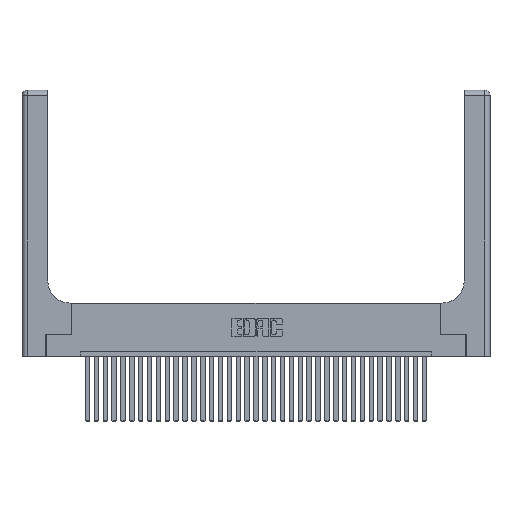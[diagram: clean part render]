
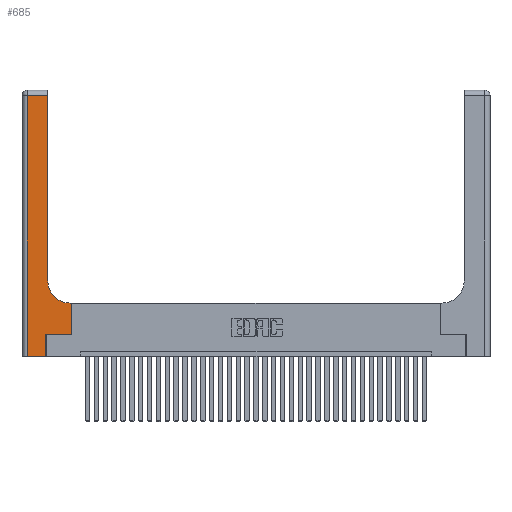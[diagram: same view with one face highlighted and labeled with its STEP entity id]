
A CAD part, top view. The second image highlights one B-rep face of the part: STEP entity #685.
In plain terms, the highlighted planar face has unit normal (0, 0, 1).
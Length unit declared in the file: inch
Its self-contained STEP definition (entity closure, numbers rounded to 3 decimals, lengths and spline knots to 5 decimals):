
#685 = ADVANCED_FACE ( 'NONE', ( #22974 ), #1935, .F. ) ;
#706 = DIRECTION ( 'NONE',  ( 1., 0., 0. ) ) ;
#1935 = PLANE ( 'NONE',  #8416 ) ;
#2700 = CARTESIAN_POINT ( 'NONE',  ( 0.269, 0.25, 0.37 ) ) ;
#2873 = VECTOR ( 'NONE', #17566, 39.37008 ) ;
#2950 = VECTOR ( 'NONE', #16315, 39.37008 ) ;
#4067 = CARTESIAN_POINT ( 'NONE',  ( 0.06, 2.94, 0.37 ) ) ;
#4298 = LINE ( 'NONE', #26759, #11896 ) ;
#4313 = LINE ( 'NONE', #32021, #24078 ) ;
#4725 = VERTEX_POINT ( 'NONE', #21585 ) ;
#5395 = VECTOR ( 'NONE', #26008, 39.37008 ) ;
#5499 = CARTESIAN_POINT ( 'NONE',  ( 0.269, 0., 0.37 ) ) ;
#6044 = VERTEX_POINT ( 'NONE', #33279 ) ;
#6497 = VERTEX_POINT ( 'NONE', #24967 ) ;
#6965 = EDGE_CURVE ( 'NONE', #30685, #6497, #4313, .T. ) ;
#8340 = EDGE_CURVE ( 'NONE', #4725, #32227, #15115, .T. ) ;
#8407 = ORIENTED_EDGE ( 'NONE', *, *, #8340, .T. ) ;
#8416 = AXIS2_PLACEMENT_3D ( 'NONE', #23293, #28463, #20472 ) ;
#8888 = EDGE_CURVE ( 'NONE', #29726, #4725, #24313, .T. ) ;
#9920 = ORIENTED_EDGE ( 'NONE', *, *, #10128, .T. ) ;
#10128 = EDGE_CURVE ( 'NONE', #32227, #30168, #34322, .T. ) ;
#10531 = VERTEX_POINT ( 'NONE', #11773 ) ;
#11012 = LINE ( 'NONE', #19578, #25315 ) ;
#11169 = DIRECTION ( 'NONE',  ( 1., 0., 0. ) ) ;
#11247 = ORIENTED_EDGE ( 'NONE', *, *, #6965, .T. ) ;
#11773 = CARTESIAN_POINT ( 'NONE',  ( 0.2915, 2.94, 0.37 ) ) ;
#11896 = VECTOR ( 'NONE', #32705, 39.37008 ) ;
#11966 = ORIENTED_EDGE ( 'NONE', *, *, #8888, .T. ) ;
#12348 = EDGE_LOOP ( 'NONE', ( #12729, #12396, #11247, #31427, #32516, #26527, #11966, #8407, #9920 ) ) ;
#12396 = ORIENTED_EDGE ( 'NONE', *, *, #17996, .T. ) ;
#12729 = ORIENTED_EDGE ( 'NONE', *, *, #33756, .T. ) ;
#12816 = CARTESIAN_POINT ( 'NONE',  ( 0.2915, 3., 0.37 ) ) ;
#13382 = DIRECTION ( 'NONE',  ( 0., 1., 0. ) ) ;
#13512 = CARTESIAN_POINT ( 'NONE',  ( 0.5415, 0.6, 0.37 ) ) ;
#14252 = CARTESIAN_POINT ( 'NONE',  ( 0.5585, 0.25, 0.37 ) ) ;
#14823 = VECTOR ( 'NONE', #13382, 39.37008 ) ;
#15115 = LINE ( 'NONE', #23066, #5395 ) ;
#16315 = DIRECTION ( 'NONE',  ( 0., 1., 0. ) ) ;
#17566 = DIRECTION ( 'NONE',  ( 0., 1., 0. ) ) ;
#17696 = CARTESIAN_POINT ( 'NONE',  ( 0.5585, 0.25, 0.37 ) ) ;
#17996 = EDGE_CURVE ( 'NONE', #10531, #30685, #4298, .T. ) ;
#19320 = LINE ( 'NONE', #5499, #2950 ) ;
#19557 = DIRECTION ( 'NONE',  ( 1., 0., 0. ) ) ;
#19578 = CARTESIAN_POINT ( 'NONE',  ( 0.269, 0.25, 0.37 ) ) ;
#19758 = CARTESIAN_POINT ( 'NONE',  ( 0.5415, 0.85, 0.37 ) ) ;
#19915 = EDGE_CURVE ( 'NONE', #6044, #21777, #19320, .T. ) ;
#20472 = DIRECTION ( 'NONE',  ( -1., 0., 0. ) ) ;
#20692 = LINE ( 'NONE', #32831, #21920 ) ;
#21003 = AXIS2_PLACEMENT_3D ( 'NONE', #19758, #26721, #11169 ) ;
#21585 = CARTESIAN_POINT ( 'NONE',  ( 0.5585, 0.6, 0.37 ) ) ;
#21777 = VERTEX_POINT ( 'NONE', #2700 ) ;
#21920 = VECTOR ( 'NONE', #19557, 39.37008 ) ;
#22329 = LINE ( 'NONE', #12816, #14823 ) ;
#22974 = FACE_OUTER_BOUND ( 'NONE', #12348, .T. ) ;
#23066 = CARTESIAN_POINT ( 'NONE',  ( 0.2915, 0.6, 0.37 ) ) ;
#23293 = CARTESIAN_POINT ( 'NONE',  ( 0., 3., 0.37 ) ) ;
#24078 = VECTOR ( 'NONE', #30248, 39.37008 ) ;
#24157 = EDGE_CURVE ( 'NONE', #21777, #29726, #11012, .T. ) ;
#24313 = LINE ( 'NONE', #17696, #2873 ) ;
#24967 = CARTESIAN_POINT ( 'NONE',  ( 0.06, 0., 0.37 ) ) ;
#25315 = VECTOR ( 'NONE', #706, 39.37008 ) ;
#26008 = DIRECTION ( 'NONE',  ( -1., 0., 0. ) ) ;
#26527 = ORIENTED_EDGE ( 'NONE', *, *, #24157, .T. ) ;
#26721 = DIRECTION ( 'NONE',  ( 0., 0., -1. ) ) ;
#26759 = CARTESIAN_POINT ( 'NONE',  ( 0., 2.94, 0.37 ) ) ;
#28463 = DIRECTION ( 'NONE',  ( 0., 0., -1. ) ) ;
#28569 = CARTESIAN_POINT ( 'NONE',  ( 0.2915, 0.85, 0.37 ) ) ;
#29726 = VERTEX_POINT ( 'NONE', #14252 ) ;
#30168 = VERTEX_POINT ( 'NONE', #28569 ) ;
#30248 = DIRECTION ( 'NONE',  ( 0., -1., 0. ) ) ;
#30685 = VERTEX_POINT ( 'NONE', #4067 ) ;
#31427 = ORIENTED_EDGE ( 'NONE', *, *, #33907, .T. ) ;
#32021 = CARTESIAN_POINT ( 'NONE',  ( 0.06, 3., 0.37 ) ) ;
#32227 = VERTEX_POINT ( 'NONE', #13512 ) ;
#32516 = ORIENTED_EDGE ( 'NONE', *, *, #19915, .T. ) ;
#32705 = DIRECTION ( 'NONE',  ( -1., 0., 0. ) ) ;
#32831 = CARTESIAN_POINT ( 'NONE',  ( 0., 0., 0.37 ) ) ;
#33279 = CARTESIAN_POINT ( 'NONE',  ( 0.269, 0., 0.37 ) ) ;
#33756 = EDGE_CURVE ( 'NONE', #30168, #10531, #22329, .T. ) ;
#33907 = EDGE_CURVE ( 'NONE', #6497, #6044, #20692, .T. ) ;
#34322 = CIRCLE ( 'NONE', #21003, 0.25 ) ;
